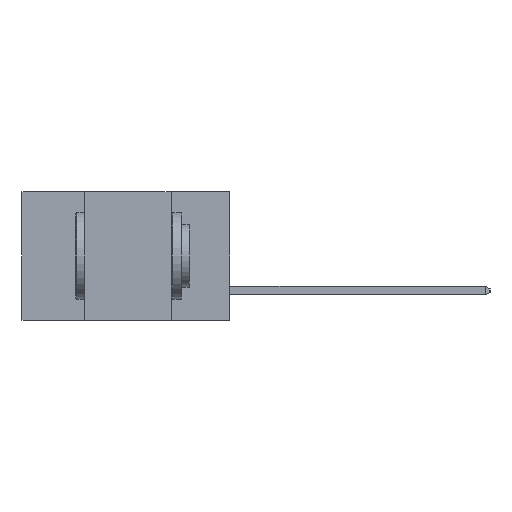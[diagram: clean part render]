
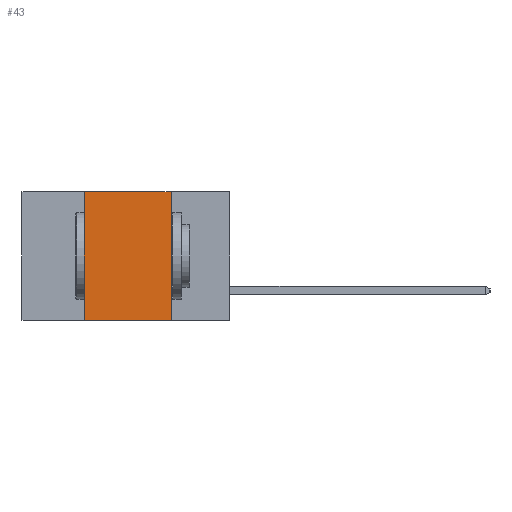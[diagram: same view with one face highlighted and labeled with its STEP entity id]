
A CAD part, left-side view. The second image highlights one B-rep face of the part: STEP entity #43.
In plain terms, the highlighted planar face has unit normal (-1, 0, 0).
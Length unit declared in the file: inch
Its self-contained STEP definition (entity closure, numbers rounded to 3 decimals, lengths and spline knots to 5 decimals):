
#43 = ADVANCED_FACE ( 'NONE', ( #1621 ), #3174, .F. ) ;
#86 = DIRECTION ( 'NONE',  ( 0., 0., -1. ) ) ;
#130 = CARTESIAN_POINT ( 'NONE',  ( 0., 0.17, -0.37 ) ) ;
#652 = VECTOR ( 'NONE', #86, 39.37008 ) ;
#746 = VERTEX_POINT ( 'NONE', #1764 ) ;
#919 = CARTESIAN_POINT ( 'NONE',  ( 0., 0.42, -0.37 ) ) ;
#1621 = FACE_OUTER_BOUND ( 'NONE', #4558, .T. ) ;
#1764 = CARTESIAN_POINT ( 'NONE',  ( 0., 0.17, -0.37 ) ) ;
#1918 = VERTEX_POINT ( 'NONE', #9812 ) ;
#2411 = ORIENTED_EDGE ( 'NONE', *, *, #5604, .F. ) ;
#3174 = PLANE ( 'NONE',  #10336 ) ;
#3265 = VECTOR ( 'NONE', #3476, 39.37008 ) ;
#3476 = DIRECTION ( 'NONE',  ( 0., -1., 0. ) ) ;
#3504 = EDGE_CURVE ( 'NONE', #1918, #746, #7240, .T. ) ;
#3555 = CARTESIAN_POINT ( 'NONE',  ( 0., 0.6, 0. ) ) ;
#4205 = DIRECTION ( 'NONE',  ( 0., 0., -1. ) ) ;
#4356 = ORIENTED_EDGE ( 'NONE', *, *, #5102, .F. ) ;
#4392 = CARTESIAN_POINT ( 'NONE',  ( 0., 0.6, 0. ) ) ;
#4403 = DIRECTION ( 'NONE',  ( 1., 0., 0. ) ) ;
#4558 = EDGE_LOOP ( 'NONE', ( #8351, #4356, #2411, #4602 ) ) ;
#4602 = ORIENTED_EDGE ( 'NONE', *, *, #7219, .T. ) ;
#5102 = EDGE_CURVE ( 'NONE', #9828, #1918, #7329, .T. ) ;
#5604 = EDGE_CURVE ( 'NONE', #8816, #9828, #8889, .T. ) ;
#5891 = VECTOR ( 'NONE', #9733, 39.37008 ) ;
#6838 = VECTOR ( 'NONE', #7614, 39.37008 ) ;
#7219 = EDGE_CURVE ( 'NONE', #8816, #746, #8257, .T. ) ;
#7240 = LINE ( 'NONE', #130, #652 ) ;
#7329 = LINE ( 'NONE', #3555, #3265 ) ;
#7614 = DIRECTION ( 'NONE',  ( 0., 0., 1. ) ) ;
#7711 = CARTESIAN_POINT ( 'NONE',  ( 0., 0.42, -0.37 ) ) ;
#8257 = LINE ( 'NONE', #9456, #5891 ) ;
#8351 = ORIENTED_EDGE ( 'NONE', *, *, #3504, .F. ) ;
#8816 = VERTEX_POINT ( 'NONE', #919 ) ;
#8889 = LINE ( 'NONE', #7711, #6838 ) ;
#9289 = CARTESIAN_POINT ( 'NONE',  ( 0., 0.42, 0. ) ) ;
#9456 = CARTESIAN_POINT ( 'NONE',  ( 0., 0.6, -0.37 ) ) ;
#9733 = DIRECTION ( 'NONE',  ( 0., -1., 0. ) ) ;
#9812 = CARTESIAN_POINT ( 'NONE',  ( 0., 0.17, 0. ) ) ;
#9828 = VERTEX_POINT ( 'NONE', #9289 ) ;
#10336 = AXIS2_PLACEMENT_3D ( 'NONE', #4392, #4403, #4205 ) ;
